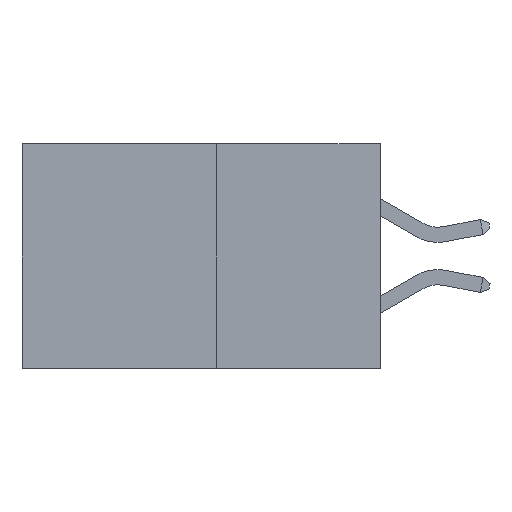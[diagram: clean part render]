
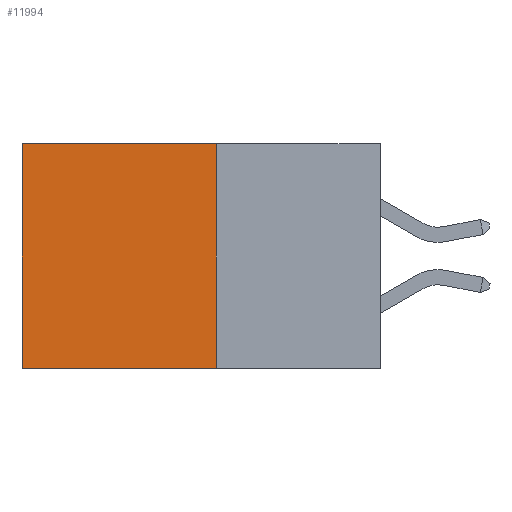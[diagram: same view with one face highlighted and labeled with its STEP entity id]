
A CAD part, left-side view. The second image highlights one B-rep face of the part: STEP entity #11994.
In plain terms, the highlighted planar face has unit normal (-1, 0, 0).
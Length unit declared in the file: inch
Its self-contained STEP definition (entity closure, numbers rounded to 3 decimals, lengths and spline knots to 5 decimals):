
#435 = EDGE_CURVE ( 'NONE', #13761, #9490, #12174, .T. ) ;
#502 = FACE_OUTER_BOUND ( 'NONE', #16822, .T. ) ;
#787 = CARTESIAN_POINT ( 'NONE',  ( 0.277, 0.27, -0.37 ) ) ;
#968 = CARTESIAN_POINT ( 'NONE',  ( 0.277, 0.27, 0. ) ) ;
#1020 = LINE ( 'NONE', #1984, #11287 ) ;
#1144 = VECTOR ( 'NONE', #16383, 39.37008 ) ;
#1342 = CARTESIAN_POINT ( 'NONE',  ( 0.277, 0.27, 0. ) ) ;
#1885 = CARTESIAN_POINT ( 'NONE',  ( 0.277, 0.59, -0.37 ) ) ;
#1984 = CARTESIAN_POINT ( 'NONE',  ( 0.277, 0.27, -0.37 ) ) ;
#2367 = VERTEX_POINT ( 'NONE', #15798 ) ;
#5650 = CARTESIAN_POINT ( 'NONE',  ( 0.277, 0.27, -0.37 ) ) ;
#6201 = DIRECTION ( 'NONE',  ( 0., 0., -1. ) ) ;
#7191 = CARTESIAN_POINT ( 'NONE',  ( 0.277, 0.59, -0.37 ) ) ;
#8272 = LINE ( 'NONE', #5650, #1144 ) ;
#8625 = VECTOR ( 'NONE', #9300, 39.37008 ) ;
#8631 = EDGE_CURVE ( 'NONE', #15170, #2367, #8272, .T. ) ;
#8669 = ORIENTED_EDGE ( 'NONE', *, *, #435, .T. ) ;
#9300 = DIRECTION ( 'NONE',  ( 0., 0., -1. ) ) ;
#9315 = AXIS2_PLACEMENT_3D ( 'NONE', #787, #14234, #6201 ) ;
#9490 = VERTEX_POINT ( 'NONE', #1885 ) ;
#11015 = CARTESIAN_POINT ( 'NONE',  ( 0.277, 0.59, 0. ) ) ;
#11174 = ORIENTED_EDGE ( 'NONE', *, *, #16984, .F. ) ;
#11287 = VECTOR ( 'NONE', #13966, 39.37008 ) ;
#11994 = ADVANCED_FACE ( 'NONE', ( #502 ), #12867, .F. ) ;
#12174 = LINE ( 'NONE', #7191, #8625 ) ;
#12867 = PLANE ( 'NONE',  #9315 ) ;
#13081 = ORIENTED_EDGE ( 'NONE', *, *, #16403, .T. ) ;
#13761 = VERTEX_POINT ( 'NONE', #11015 ) ;
#13966 = DIRECTION ( 'NONE',  ( 0., 1., 0. ) ) ;
#14234 = DIRECTION ( 'NONE',  ( 1., 0., 0. ) ) ;
#14343 = DIRECTION ( 'NONE',  ( 0., 1., 0. ) ) ;
#15170 = VERTEX_POINT ( 'NONE', #1342 ) ;
#15798 = CARTESIAN_POINT ( 'NONE',  ( 0.277, 0.27, -0.37 ) ) ;
#16282 = ORIENTED_EDGE ( 'NONE', *, *, #8631, .F. ) ;
#16383 = DIRECTION ( 'NONE',  ( 0., 0., -1. ) ) ;
#16403 = EDGE_CURVE ( 'NONE', #15170, #13761, #16593, .T. ) ;
#16593 = LINE ( 'NONE', #968, #16993 ) ;
#16822 = EDGE_LOOP ( 'NONE', ( #8669, #11174, #16282, #13081 ) ) ;
#16984 = EDGE_CURVE ( 'NONE', #2367, #9490, #1020, .T. ) ;
#16993 = VECTOR ( 'NONE', #14343, 39.37008 ) ;
